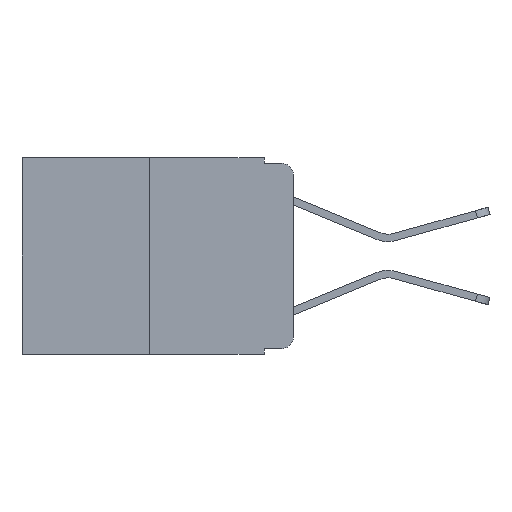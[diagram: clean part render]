
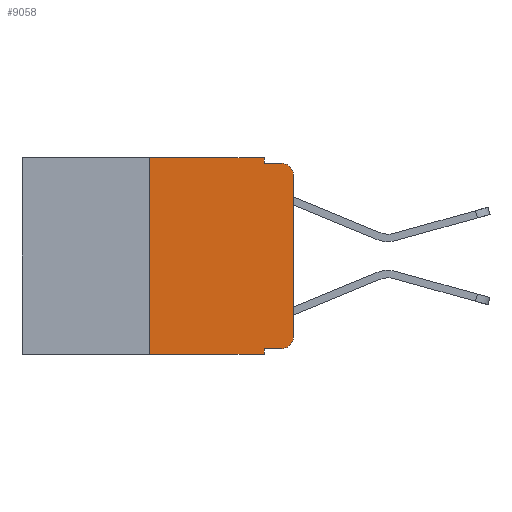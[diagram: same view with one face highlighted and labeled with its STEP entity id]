
A CAD part, left-side view. The second image highlights one B-rep face of the part: STEP entity #9058.
In plain terms, the highlighted planar face has unit normal (-1, 0, 0).
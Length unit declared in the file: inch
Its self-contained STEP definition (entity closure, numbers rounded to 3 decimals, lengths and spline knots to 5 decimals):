
#216 = PLANE ( 'NONE',  #8373 ) ;
#427 = CARTESIAN_POINT ( 'NONE',  ( 0., 0., -0.313 ) ) ;
#509 = VECTOR ( 'NONE', #5178, 39.37008 ) ;
#514 = CARTESIAN_POINT ( 'NONE',  ( 0., 0.051, -0.01 ) ) ;
#643 = DIRECTION ( 'NONE',  ( 0., -1., 0. ) ) ;
#704 = EDGE_CURVE ( 'NONE', #1024, #2953, #1134, .T. ) ;
#912 = ORIENTED_EDGE ( 'NONE', *, *, #1506, .F. ) ;
#1024 = VERTEX_POINT ( 'NONE', #11506 ) ;
#1134 = LINE ( 'NONE', #1172, #3617 ) ;
#1172 = CARTESIAN_POINT ( 'NONE',  ( 0., 0.25, 0. ) ) ;
#1296 = VECTOR ( 'NONE', #8674, 39.37008 ) ;
#1506 = EDGE_CURVE ( 'NONE', #2426, #8654, #7284, .T. ) ;
#2068 = CARTESIAN_POINT ( 'NONE',  ( 0., 0.051, 0. ) ) ;
#2229 = EDGE_CURVE ( 'NONE', #8654, #12905, #9244, .T. ) ;
#2275 = DIRECTION ( 'NONE',  ( 0., 0., -1. ) ) ;
#2297 = ORIENTED_EDGE ( 'NONE', *, *, #3428, .F. ) ;
#2343 = CARTESIAN_POINT ( 'NONE',  ( 0., 0.051, -0.343 ) ) ;
#2426 = VERTEX_POINT ( 'NONE', #10193 ) ;
#2511 = AXIS2_PLACEMENT_3D ( 'NONE', #3461, #10289, #4444 ) ;
#2524 = CARTESIAN_POINT ( 'NONE',  ( 0., 0.473, 0. ) ) ;
#2542 = LINE ( 'NONE', #10215, #7818 ) ;
#2953 = VERTEX_POINT ( 'NONE', #12849 ) ;
#3028 = CARTESIAN_POINT ( 'NONE',  ( 0., 0.051, 0. ) ) ;
#3295 = CARTESIAN_POINT ( 'NONE',  ( 0., 0., -0.03 ) ) ;
#3309 = DIRECTION ( 'NONE',  ( -1., 0., 0. ) ) ;
#3428 = EDGE_CURVE ( 'NONE', #2953, #2426, #4960, .T. ) ;
#3461 = CARTESIAN_POINT ( 'NONE',  ( 0., 0.02, -0.313 ) ) ;
#3617 = VECTOR ( 'NONE', #6832, 39.37008 ) ;
#4101 = CARTESIAN_POINT ( 'NONE',  ( 0., 0.051, -0.333 ) ) ;
#4375 = DIRECTION ( 'NONE',  ( 0., -1., 0. ) ) ;
#4444 = DIRECTION ( 'NONE',  ( 0., 0., -1. ) ) ;
#4638 = VECTOR ( 'NONE', #2275, 39.37008 ) ;
#4915 = VERTEX_POINT ( 'NONE', #8629 ) ;
#4960 = LINE ( 'NONE', #12586, #9843 ) ;
#5178 = DIRECTION ( 'NONE',  ( 0., 0., 1. ) ) ;
#5310 = CIRCLE ( 'NONE', #2511, 0.02 ) ;
#5376 = DIRECTION ( 'NONE',  ( 0., -1., 0. ) ) ;
#5393 = ORIENTED_EDGE ( 'NONE', *, *, #2229, .F. ) ;
#6233 = EDGE_CURVE ( 'NONE', #6931, #12905, #12535, .T. ) ;
#6341 = LINE ( 'NONE', #11972, #509 ) ;
#6393 = LINE ( 'NONE', #11178, #8975 ) ;
#6485 = ORIENTED_EDGE ( 'NONE', *, *, #10361, .T. ) ;
#6514 = DIRECTION ( 'NONE',  ( 0., 0., -1. ) ) ;
#6832 = DIRECTION ( 'NONE',  ( 0., 0., 1. ) ) ;
#6900 = EDGE_CURVE ( 'NONE', #9834, #6931, #6341, .T. ) ;
#6931 = VERTEX_POINT ( 'NONE', #3295 ) ;
#7284 = LINE ( 'NONE', #2068, #4638 ) ;
#7367 = AXIS2_PLACEMENT_3D ( 'NONE', #9159, #3309, #10128 ) ;
#7568 = VECTOR ( 'NONE', #7950, 39.37008 ) ;
#7818 = VECTOR ( 'NONE', #4375, 39.37008 ) ;
#7950 = DIRECTION ( 'NONE',  ( 0., 0., -1. ) ) ;
#8068 = ORIENTED_EDGE ( 'NONE', *, *, #704, .F. ) ;
#8299 = ORIENTED_EDGE ( 'NONE', *, *, #10993, .T. ) ;
#8373 = AXIS2_PLACEMENT_3D ( 'NONE', #2524, #12296, #6514 ) ;
#8446 = ORIENTED_EDGE ( 'NONE', *, *, #6900, .T. ) ;
#8629 = CARTESIAN_POINT ( 'NONE',  ( 0., 0.02, -0.333 ) ) ;
#8654 = VERTEX_POINT ( 'NONE', #514 ) ;
#8674 = DIRECTION ( 'NONE',  ( 0., -1., 0. ) ) ;
#8701 = CARTESIAN_POINT ( 'NONE',  ( 0., 0.051, -0.01 ) ) ;
#8741 = ORIENTED_EDGE ( 'NONE', *, *, #6233, .T. ) ;
#8975 = VECTOR ( 'NONE', #5376, 39.37008 ) ;
#9058 = ADVANCED_FACE ( 'NONE', ( #10964 ), #216, .F. ) ;
#9159 = CARTESIAN_POINT ( 'NONE',  ( 0., 0.02, -0.03 ) ) ;
#9244 = LINE ( 'NONE', #8701, #1296 ) ;
#9640 = EDGE_CURVE ( 'NONE', #1024, #10959, #2542, .T. ) ;
#9834 = VERTEX_POINT ( 'NONE', #427 ) ;
#9843 = VECTOR ( 'NONE', #643, 39.37008 ) ;
#10128 = DIRECTION ( 'NONE',  ( 0., 0., -1. ) ) ;
#10129 = VERTEX_POINT ( 'NONE', #4101 ) ;
#10193 = CARTESIAN_POINT ( 'NONE',  ( 0., 0.051, 0. ) ) ;
#10215 = CARTESIAN_POINT ( 'NONE',  ( 0., 0.473, -0.343 ) ) ;
#10289 = DIRECTION ( 'NONE',  ( -1., 0., 0. ) ) ;
#10361 = EDGE_CURVE ( 'NONE', #4915, #9834, #5310, .T. ) ;
#10870 = EDGE_LOOP ( 'NONE', ( #8446, #8741, #5393, #912, #2297, #8068, #11020, #11445, #8299, #6485 ) ) ;
#10959 = VERTEX_POINT ( 'NONE', #2343 ) ;
#10964 = FACE_OUTER_BOUND ( 'NONE', #10870, .T. ) ;
#10993 = EDGE_CURVE ( 'NONE', #10129, #4915, #6393, .T. ) ;
#11020 = ORIENTED_EDGE ( 'NONE', *, *, #9640, .T. ) ;
#11178 = CARTESIAN_POINT ( 'NONE',  ( 0., 0.051, -0.333 ) ) ;
#11445 = ORIENTED_EDGE ( 'NONE', *, *, #12947, .F. ) ;
#11506 = CARTESIAN_POINT ( 'NONE',  ( 0., 0.25, -0.343 ) ) ;
#11972 = CARTESIAN_POINT ( 'NONE',  ( 0., 0., 0. ) ) ;
#12296 = DIRECTION ( 'NONE',  ( 1., 0., 0. ) ) ;
#12535 = CIRCLE ( 'NONE', #7367, 0.02 ) ;
#12586 = CARTESIAN_POINT ( 'NONE',  ( 0., 0.473, 0. ) ) ;
#12674 = LINE ( 'NONE', #3028, #7568 ) ;
#12698 = CARTESIAN_POINT ( 'NONE',  ( 0., 0.02, -0.01 ) ) ;
#12849 = CARTESIAN_POINT ( 'NONE',  ( 0., 0.25, 0. ) ) ;
#12905 = VERTEX_POINT ( 'NONE', #12698 ) ;
#12947 = EDGE_CURVE ( 'NONE', #10129, #10959, #12674, .T. ) ;
